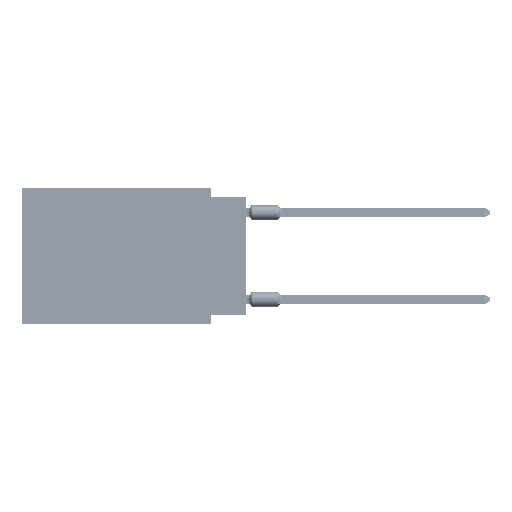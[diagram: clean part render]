
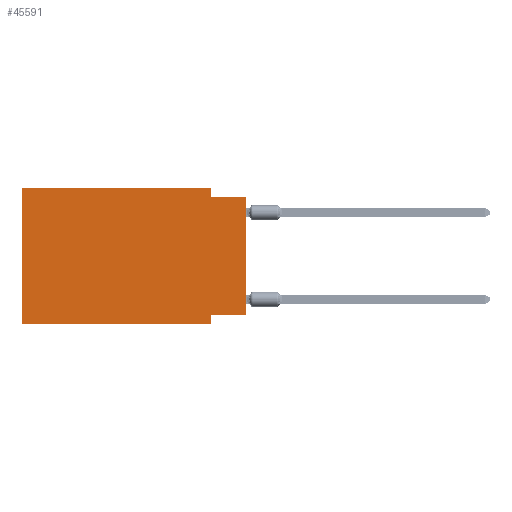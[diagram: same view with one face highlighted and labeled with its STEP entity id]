
A CAD part, left-side view. The second image highlights one B-rep face of the part: STEP entity #45591.
In plain terms, the highlighted planar face has unit normal (-1, 0, 0).
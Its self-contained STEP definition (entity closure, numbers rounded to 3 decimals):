
#2494 = CARTESIAN_POINT ( 'NONE',  ( 0., 0., -0.635 ) ) ;
#3275 = LINE ( 'NONE', #13877, #55491 ) ;
#4653 = DIRECTION ( 'NONE',  ( 1., 0., 0. ) ) ;
#6536 = EDGE_CURVE ( 'NONE', #64311, #59277, #35434, .T. ) ;
#8065 = DIRECTION ( 'NONE',  ( 0., 0., 1. ) ) ;
#8858 = VERTEX_POINT ( 'NONE', #29172 ) ;
#9787 = CARTESIAN_POINT ( 'NONE',  ( 0., 16.383, 0. ) ) ;
#11410 = EDGE_CURVE ( 'NONE', #21417, #19525, #3275, .T. ) ;
#13877 = CARTESIAN_POINT ( 'NONE',  ( 0., 16.383, 0. ) ) ;
#13926 = CARTESIAN_POINT ( 'NONE',  ( 0., 16.383, 0. ) ) ;
#18382 = EDGE_CURVE ( 'NONE', #20797, #64826, #47760, .T. ) ;
#19525 = VERTEX_POINT ( 'NONE', #46105 ) ;
#19605 = LINE ( 'NONE', #66806, #37978 ) ;
#20797 = VERTEX_POINT ( 'NONE', #24946 ) ;
#21417 = VERTEX_POINT ( 'NONE', #24034 ) ;
#22921 = CARTESIAN_POINT ( 'NONE',  ( 0., 2.54, 0. ) ) ;
#24034 = CARTESIAN_POINT ( 'NONE',  ( 0., 16.383, -9.906 ) ) ;
#24946 = CARTESIAN_POINT ( 'NONE',  ( 0., 0., -9.271 ) ) ;
#25515 = DIRECTION ( 'NONE',  ( 0., 0., -1. ) ) ;
#25676 = LINE ( 'NONE', #67408, #41018 ) ;
#29172 = CARTESIAN_POINT ( 'NONE',  ( 0., 0., -0.635 ) ) ;
#29447 = VECTOR ( 'NONE', #54493, 1000. ) ;
#31280 = EDGE_CURVE ( 'NONE', #21417, #53454, #19605, .T. ) ;
#32305 = AXIS2_PLACEMENT_3D ( 'NONE', #9787, #4653, #25515 ) ;
#32446 = EDGE_CURVE ( 'NONE', #19525, #64311, #60122, .T. ) ;
#32919 = VECTOR ( 'NONE', #36187, 1000. ) ;
#33042 = ORIENTED_EDGE ( 'NONE', *, *, #32446, .F. ) ;
#33106 = ORIENTED_EDGE ( 'NONE', *, *, #53037, .T. ) ;
#34602 = ORIENTED_EDGE ( 'NONE', *, *, #11410, .F. ) ;
#35434 = LINE ( 'NONE', #56299, #67344 ) ;
#36187 = DIRECTION ( 'NONE',  ( 0., 0., 1. ) ) ;
#37017 = CARTESIAN_POINT ( 'NONE',  ( 0., 2.54, -0.635 ) ) ;
#37978 = VECTOR ( 'NONE', #41824, 1000. ) ;
#38052 = ORIENTED_EDGE ( 'NONE', *, *, #44796, .F. ) ;
#38493 = VECTOR ( 'NONE', #57040, 1000. ) ;
#40266 = ORIENTED_EDGE ( 'NONE', *, *, #31280, .T. ) ;
#40597 = ORIENTED_EDGE ( 'NONE', *, *, #6536, .F. ) ;
#41018 = VECTOR ( 'NONE', #62300, 1000. ) ;
#41824 = DIRECTION ( 'NONE',  ( 0., -1., 0. ) ) ;
#41988 = CARTESIAN_POINT ( 'NONE',  ( 0., 0., 0. ) ) ;
#44796 = EDGE_CURVE ( 'NONE', #64826, #53454, #25676, .T. ) ;
#45591 = ADVANCED_FACE ( 'NONE', ( #61789 ), #56662, .F. ) ;
#46105 = CARTESIAN_POINT ( 'NONE',  ( 0., 16.383, 0. ) ) ;
#47760 = LINE ( 'NONE', #63505, #38493 ) ;
#47926 = VECTOR ( 'NONE', #66598, 1000. ) ;
#51845 = CARTESIAN_POINT ( 'NONE',  ( 0., 2.54, -9.906 ) ) ;
#53037 = EDGE_CURVE ( 'NONE', #20797, #8858, #57736, .T. ) ;
#53454 = VERTEX_POINT ( 'NONE', #51845 ) ;
#54493 = DIRECTION ( 'NONE',  ( 0., -1., 0. ) ) ;
#55491 = VECTOR ( 'NONE', #8065, 1000. ) ;
#56299 = CARTESIAN_POINT ( 'NONE',  ( 0., 2.54, 0. ) ) ;
#56662 = PLANE ( 'NONE',  #32305 ) ;
#57040 = DIRECTION ( 'NONE',  ( 0., 1., 0. ) ) ;
#57736 = LINE ( 'NONE', #41988, #32919 ) ;
#59202 = EDGE_LOOP ( 'NONE', ( #33106, #60176, #40597, #33042, #34602, #40266, #38052, #64647 ) ) ;
#59277 = VERTEX_POINT ( 'NONE', #37017 ) ;
#60122 = LINE ( 'NONE', #13926, #47926 ) ;
#60176 = ORIENTED_EDGE ( 'NONE', *, *, #66092, .F. ) ;
#61776 = DIRECTION ( 'NONE',  ( 0., 0., -1. ) ) ;
#61789 = FACE_OUTER_BOUND ( 'NONE', #59202, .T. ) ;
#62300 = DIRECTION ( 'NONE',  ( 0., 0., -1. ) ) ;
#62817 = LINE ( 'NONE', #2494, #29447 ) ;
#63505 = CARTESIAN_POINT ( 'NONE',  ( 0., 0., -9.271 ) ) ;
#64311 = VERTEX_POINT ( 'NONE', #22921 ) ;
#64415 = CARTESIAN_POINT ( 'NONE',  ( 0., 2.54, -9.271 ) ) ;
#64647 = ORIENTED_EDGE ( 'NONE', *, *, #18382, .F. ) ;
#64826 = VERTEX_POINT ( 'NONE', #64415 ) ;
#66092 = EDGE_CURVE ( 'NONE', #59277, #8858, #62817, .T. ) ;
#66598 = DIRECTION ( 'NONE',  ( 0., -1., 0. ) ) ;
#66806 = CARTESIAN_POINT ( 'NONE',  ( 0., 16.383, -9.906 ) ) ;
#67344 = VECTOR ( 'NONE', #61776, 1000. ) ;
#67408 = CARTESIAN_POINT ( 'NONE',  ( 0., 2.54, -9.906 ) ) ;
